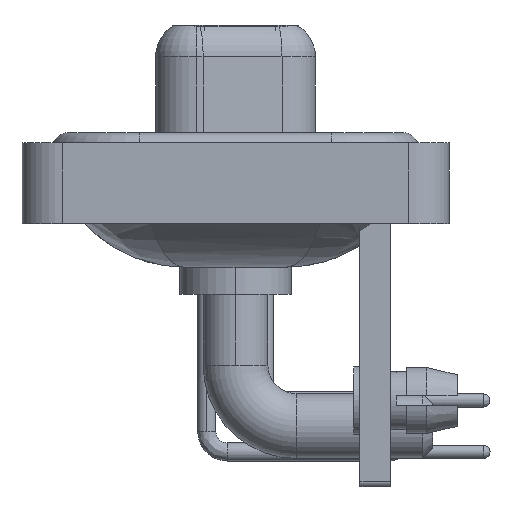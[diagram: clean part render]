
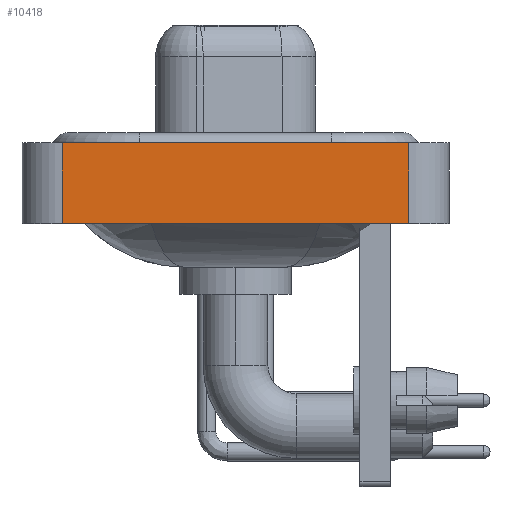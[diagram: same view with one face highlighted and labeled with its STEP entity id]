
A CAD part, left-side view. The second image highlights one B-rep face of the part: STEP entity #10418.
In plain terms, the highlighted planar face has unit normal (-1, 0, 0).
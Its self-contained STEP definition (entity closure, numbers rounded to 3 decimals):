
#714 = EDGE_CURVE ( 'NONE', #20923, #21455, #3752, .T. ) ;
#2044 = LINE ( 'NONE', #10272, #7469 ) ;
#2711 = DIRECTION ( 'NONE',  ( -1., 0., 0. ) ) ;
#2926 = ORIENTED_EDGE ( 'NONE', *, *, #714, .F. ) ;
#3752 = LINE ( 'NONE', #7726, #17924 ) ;
#4916 = PLANE ( 'NONE',  #13186 ) ;
#6704 = FACE_OUTER_BOUND ( 'NONE', #25985, .T. ) ;
#6871 = VERTEX_POINT ( 'NONE', #13713 ) ;
#7469 = VECTOR ( 'NONE', #18651, 1000. ) ;
#7726 = CARTESIAN_POINT ( 'NONE',  ( -7.35, -8.55, 0.4 ) ) ;
#9045 = VERTEX_POINT ( 'NONE', #14175 ) ;
#10272 = CARTESIAN_POINT ( 'NONE',  ( -7.35, -8.55, -3.6 ) ) ;
#10418 = ADVANCED_FACE ( 'NONE', ( #6704 ), #4916, .T. ) ;
#10634 = ORIENTED_EDGE ( 'NONE', *, *, #20733, .T. ) ;
#10665 = EDGE_CURVE ( 'NONE', #6871, #21455, #20808, .T. ) ;
#12015 = DIRECTION ( 'NONE',  ( 0., 0., 1. ) ) ;
#12868 = CARTESIAN_POINT ( 'NONE',  ( -7.35, -8.55, -3.6 ) ) ;
#13186 = AXIS2_PLACEMENT_3D ( 'NONE', #12868, #2711, #21109 ) ;
#13713 = CARTESIAN_POINT ( 'NONE',  ( -7.35, -8.55, -3.6 ) ) ;
#14020 = CARTESIAN_POINT ( 'NONE',  ( -7.35, -8.55, 0.4 ) ) ;
#14175 = CARTESIAN_POINT ( 'NONE',  ( -7.35, 8.55, -3.6 ) ) ;
#16089 = DIRECTION ( 'NONE',  ( 0., 0., 1. ) ) ;
#17152 = ORIENTED_EDGE ( 'NONE', *, *, #23244, .F. ) ;
#17388 = CARTESIAN_POINT ( 'NONE',  ( -7.35, 8.55, 0.4 ) ) ;
#17745 = LINE ( 'NONE', #24209, #20349 ) ;
#17924 = VECTOR ( 'NONE', #20362, 1000. ) ;
#18651 = DIRECTION ( 'NONE',  ( 0., -1., 0. ) ) ;
#20349 = VECTOR ( 'NONE', #16089, 1000. ) ;
#20362 = DIRECTION ( 'NONE',  ( 0., -1., 0. ) ) ;
#20733 = EDGE_CURVE ( 'NONE', #9045, #6871, #2044, .T. ) ;
#20808 = LINE ( 'NONE', #27126, #23752 ) ;
#20923 = VERTEX_POINT ( 'NONE', #17388 ) ;
#21109 = DIRECTION ( 'NONE',  ( 0., 0., 1. ) ) ;
#21455 = VERTEX_POINT ( 'NONE', #14020 ) ;
#23244 = EDGE_CURVE ( 'NONE', #9045, #20923, #17745, .T. ) ;
#23752 = VECTOR ( 'NONE', #12015, 1000. ) ;
#24209 = CARTESIAN_POINT ( 'NONE',  ( -7.35, 8.55, -3.6 ) ) ;
#25985 = EDGE_LOOP ( 'NONE', ( #26901, #2926, #17152, #10634 ) ) ;
#26901 = ORIENTED_EDGE ( 'NONE', *, *, #10665, .T. ) ;
#27126 = CARTESIAN_POINT ( 'NONE',  ( -7.35, -8.55, -3.6 ) ) ;
